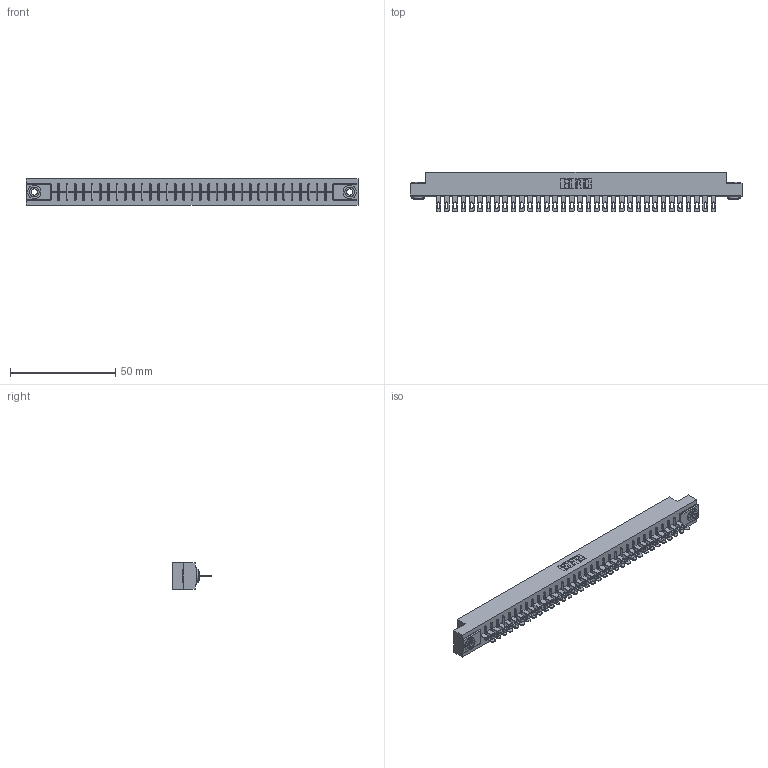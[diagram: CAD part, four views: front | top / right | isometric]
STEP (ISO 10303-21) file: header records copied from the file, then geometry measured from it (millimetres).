
FILE_DESCRIPTION (( 'STEP AP203' ), '1' );
FILE_NAME ('356-034-500-103.STEP', '2018-08-01T21:30:29', ( '' ), ( '' ), 'SwSTEP 2.0', 'SolidWorks 2016', '' );
FILE_SCHEMA (( 'CONFIG_CONTROL_DESIGN' ));
Length unit declared in the file: inch
Products named in the file (4): 306 Part_.156 Dia; 306-290-001_100; 345-250-002_345-250-002-102; 356-034-500-103
Assembly tree (37 placements, depth 2):
  356-034-500-103
    306 Part_.156 Dia
    306-290-001_100  x34
    345-250-002_345-250-002-102  x2
Bounding box: 157.73 x 18.87 x 12.7 mm (x, y, z)
Volume: 17479.5 mm3; surface area: 18711.7 mm2
Topology: 37 solids, 37 shells, 2752 faces, 7738 edges, 4972 vertices
Faces by surface type: plane 1792, cylinder 816, sphere 136, cone 8
Entity records: 33972 total; most frequent: CARTESIAN_POINT 5682, ORIENTED_EDGE 5624, DIRECTION 5618, EDGE_CURVE 2812, LINE 2186, VECTOR 2186, VERTEX_POINT 1780, AXIS2_PLACEMENT_3D 1716
